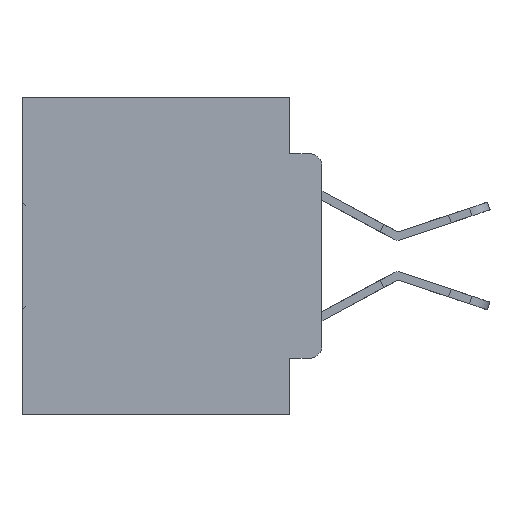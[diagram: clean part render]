
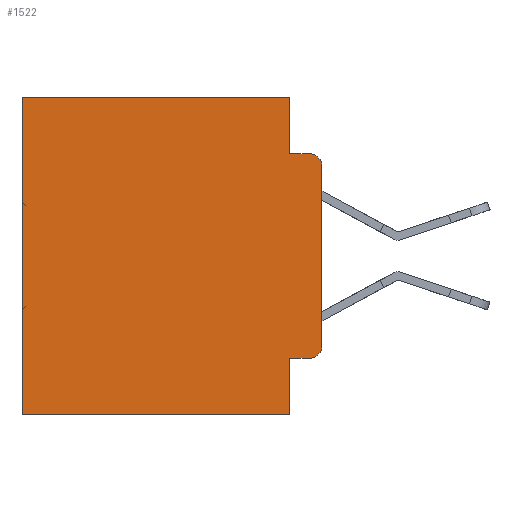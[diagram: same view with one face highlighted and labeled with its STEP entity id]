
A CAD part, left-side view. The second image highlights one B-rep face of the part: STEP entity #1522.
In plain terms, the highlighted planar face has unit normal (-1, 0, 0).
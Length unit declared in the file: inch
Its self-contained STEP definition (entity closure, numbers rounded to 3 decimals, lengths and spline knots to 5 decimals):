
#1079 = EDGE_CURVE ( 'NONE', #30440, #32677, #5961, .T. ) ;
#1186 = CIRCLE ( 'NONE', #31545, 0.02 ) ;
#1522 = ADVANCED_FACE ( 'NONE', ( #12131 ), #5822, .F. ) ;
#2071 = VECTOR ( 'NONE', #29892, 39.37008 ) ;
#2288 = DIRECTION ( 'NONE',  ( 0., 1., 0. ) ) ;
#2576 = CARTESIAN_POINT ( 'NONE',  ( 0.298, 0., -0.3915 ) ) ;
#2591 = VERTEX_POINT ( 'NONE', #9455 ) ;
#2946 = DIRECTION ( 'NONE',  ( 0., 1., 0. ) ) ;
#2986 = ORIENTED_EDGE ( 'NONE', *, *, #8429, .F. ) ;
#4268 = LINE ( 'NONE', #18818, #32193 ) ;
#4686 = LINE ( 'NONE', #27164, #31806 ) ;
#4923 = EDGE_CURVE ( 'NONE', #30440, #5188, #8716, .T. ) ;
#5184 = EDGE_CURVE ( 'NONE', #2591, #32677, #1186, .T. ) ;
#5188 = VERTEX_POINT ( 'NONE', #19097 ) ;
#5387 = EDGE_CURVE ( 'NONE', #12022, #2591, #23213, .T. ) ;
#5790 = CARTESIAN_POINT ( 'NONE',  ( 0.298, 0., 0. ) ) ;
#5822 = PLANE ( 'NONE',  #28409 ) ;
#5961 = LINE ( 'NONE', #23934, #12994 ) ;
#6080 = LINE ( 'NONE', #7546, #19292 ) ;
#7125 = ORIENTED_EDGE ( 'NONE', *, *, #4923, .T. ) ;
#7546 = CARTESIAN_POINT ( 'NONE',  ( 0.298, 0.051, -0.0885 ) ) ;
#8159 = CARTESIAN_POINT ( 'NONE',  ( 0.298, 0.051, 0. ) ) ;
#8429 = EDGE_CURVE ( 'NONE', #10903, #5188, #6080, .T. ) ;
#8716 = CIRCLE ( 'NONE', #32176, 0.02 ) ;
#8842 = ORIENTED_EDGE ( 'NONE', *, *, #28963, .T. ) ;
#9455 = CARTESIAN_POINT ( 'NONE',  ( 0.298, 0.02, -0.4115 ) ) ;
#9775 = VERTEX_POINT ( 'NONE', #26135 ) ;
#10201 = DIRECTION ( 'NONE',  ( 0., -1., 0. ) ) ;
#10376 = CARTESIAN_POINT ( 'NONE',  ( 0.298, 0.473, 0. ) ) ;
#10839 = DIRECTION ( 'NONE',  ( 0., 0., -1. ) ) ;
#10903 = VERTEX_POINT ( 'NONE', #20878 ) ;
#11790 = ORIENTED_EDGE ( 'NONE', *, *, #18441, .F. ) ;
#11839 = VECTOR ( 'NONE', #2288, 39.37008 ) ;
#12022 = VERTEX_POINT ( 'NONE', #12716 ) ;
#12131 = FACE_OUTER_BOUND ( 'NONE', #21994, .T. ) ;
#12403 = VECTOR ( 'NONE', #32989, 39.37008 ) ;
#12622 = DIRECTION ( 'NONE',  ( 1., 0., 0. ) ) ;
#12651 = DIRECTION ( 'NONE',  ( 0., 0., -1. ) ) ;
#12716 = CARTESIAN_POINT ( 'NONE',  ( 0.298, 0.051, -0.4115 ) ) ;
#12772 = LINE ( 'NONE', #8159, #25975 ) ;
#12866 = CARTESIAN_POINT ( 'NONE',  ( 0.298, 0.051, -0.5 ) ) ;
#12994 = VECTOR ( 'NONE', #27477, 39.37008 ) ;
#13467 = ORIENTED_EDGE ( 'NONE', *, *, #5387, .T. ) ;
#14680 = CARTESIAN_POINT ( 'NONE',  ( 0.298, 0.473, 0. ) ) ;
#16360 = ORIENTED_EDGE ( 'NONE', *, *, #5184, .T. ) ;
#16568 = CARTESIAN_POINT ( 'NONE',  ( 0.298, 0.473, -0.5 ) ) ;
#17525 = ORIENTED_EDGE ( 'NONE', *, *, #20864, .F. ) ;
#18441 = EDGE_CURVE ( 'NONE', #12022, #26703, #4686, .T. ) ;
#18818 = CARTESIAN_POINT ( 'NONE',  ( 0.298, 0., 0. ) ) ;
#18931 = VERTEX_POINT ( 'NONE', #10376 ) ;
#19093 = CARTESIAN_POINT ( 'NONE',  ( 0.298, 0.02, -0.3915 ) ) ;
#19097 = CARTESIAN_POINT ( 'NONE',  ( 0.298, 0.02, -0.0885 ) ) ;
#19292 = VECTOR ( 'NONE', #10201, 39.37008 ) ;
#19363 = DIRECTION ( 'NONE',  ( 0., 0., -1. ) ) ;
#19474 = DIRECTION ( 'NONE',  ( 0., 0., -1. ) ) ;
#19786 = DIRECTION ( 'NONE',  ( -1., 0., 0. ) ) ;
#20303 = ORIENTED_EDGE ( 'NONE', *, *, #1079, .F. ) ;
#20835 = ORIENTED_EDGE ( 'NONE', *, *, #27514, .T. ) ;
#20864 = EDGE_CURVE ( 'NONE', #9775, #10903, #12772, .T. ) ;
#20878 = CARTESIAN_POINT ( 'NONE',  ( 0.298, 0.051, -0.0885 ) ) ;
#21007 = VERTEX_POINT ( 'NONE', #16568 ) ;
#21994 = EDGE_LOOP ( 'NONE', ( #20303, #7125, #2986, #17525, #20835, #8842, #28645, #11790, #13467, #16360 ) ) ;
#23213 = LINE ( 'NONE', #27241, #2071 ) ;
#23367 = CARTESIAN_POINT ( 'NONE',  ( 0.298, 0., -0.5 ) ) ;
#23934 = CARTESIAN_POINT ( 'NONE',  ( 0.298, 0., 0. ) ) ;
#24848 = EDGE_CURVE ( 'NONE', #26703, #21007, #32747, .T. ) ;
#25975 = VECTOR ( 'NONE', #10839, 39.37008 ) ;
#26135 = CARTESIAN_POINT ( 'NONE',  ( 0.298, 0.051, 0. ) ) ;
#26414 = LINE ( 'NONE', #14680, #12403 ) ;
#26703 = VERTEX_POINT ( 'NONE', #12866 ) ;
#27094 = CARTESIAN_POINT ( 'NONE',  ( 0.298, 0., -0.1085 ) ) ;
#27164 = CARTESIAN_POINT ( 'NONE',  ( 0.298, 0.051, 0. ) ) ;
#27241 = CARTESIAN_POINT ( 'NONE',  ( 0.298, 0.051, -0.4115 ) ) ;
#27477 = DIRECTION ( 'NONE',  ( 0., 0., -1. ) ) ;
#27514 = EDGE_CURVE ( 'NONE', #9775, #18931, #4268, .T. ) ;
#28278 = DIRECTION ( 'NONE',  ( -1., 0., 0. ) ) ;
#28321 = CARTESIAN_POINT ( 'NONE',  ( 0.298, 0.02, -0.1085 ) ) ;
#28409 = AXIS2_PLACEMENT_3D ( 'NONE', #5790, #12622, #12651 ) ;
#28475 = DIRECTION ( 'NONE',  ( 0., 0., -1. ) ) ;
#28645 = ORIENTED_EDGE ( 'NONE', *, *, #24848, .F. ) ;
#28963 = EDGE_CURVE ( 'NONE', #18931, #21007, #26414, .T. ) ;
#29892 = DIRECTION ( 'NONE',  ( 0., -1., 0. ) ) ;
#30440 = VERTEX_POINT ( 'NONE', #27094 ) ;
#31545 = AXIS2_PLACEMENT_3D ( 'NONE', #19093, #19786, #19474 ) ;
#31806 = VECTOR ( 'NONE', #19363, 39.37008 ) ;
#32176 = AXIS2_PLACEMENT_3D ( 'NONE', #28321, #28278, #28475 ) ;
#32193 = VECTOR ( 'NONE', #2946, 39.37008 ) ;
#32677 = VERTEX_POINT ( 'NONE', #2576 ) ;
#32747 = LINE ( 'NONE', #23367, #11839 ) ;
#32989 = DIRECTION ( 'NONE',  ( 0., 0., -1. ) ) ;
